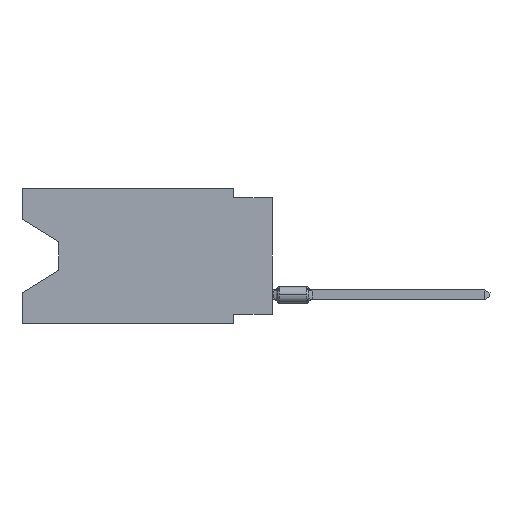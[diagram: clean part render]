
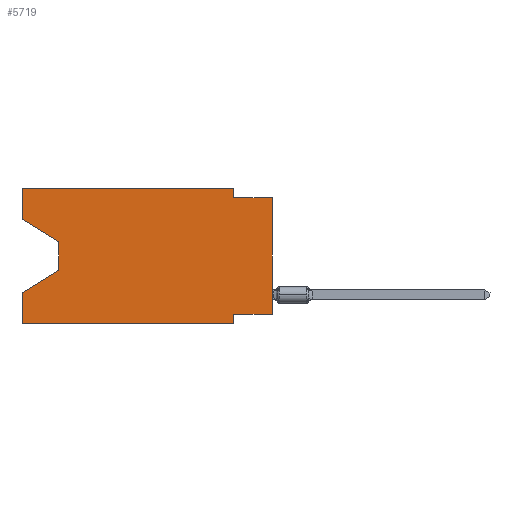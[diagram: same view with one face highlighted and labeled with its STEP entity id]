
A CAD part, left-side view. The second image highlights one B-rep face of the part: STEP entity #5719.
In plain terms, the highlighted planar face has unit normal (-1, 0, 0).
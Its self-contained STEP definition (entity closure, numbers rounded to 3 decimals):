
#72 = ORIENTED_EDGE ( 'NONE', *, *, #1886, .T. ) ;
#1260 = EDGE_CURVE ( 'NONE', #10910, #20803, #10194, .T. ) ;
#1364 = ORIENTED_EDGE ( 'NONE', *, *, #1512, .F. ) ;
#1512 = EDGE_CURVE ( 'NONE', #18159, #8420, #3695, .T. ) ;
#1534 = CARTESIAN_POINT ( 'NONE',  ( 0., 2.54, 0. ) ) ;
#1568 = ORIENTED_EDGE ( 'NONE', *, *, #5240, .T. ) ;
#1886 = EDGE_CURVE ( 'NONE', #2722, #25753, #18234, .T. ) ;
#1887 = VECTOR ( 'NONE', #8162, 1000. ) ;
#2142 = DIRECTION ( 'NONE',  ( 0., 0., 1. ) ) ;
#2150 = DIRECTION ( 'NONE',  ( 0., 0., -1. ) ) ;
#2157 = ORIENTED_EDGE ( 'NONE', *, *, #17376, .F. ) ;
#2531 = VERTEX_POINT ( 'NONE', #14428 ) ;
#2722 = VERTEX_POINT ( 'NONE', #5705 ) ;
#3095 = EDGE_CURVE ( 'NONE', #8420, #15817, #4840, .T. ) ;
#3123 = EDGE_CURVE ( 'NONE', #20083, #2722, #16212, .T. ) ;
#3695 = LINE ( 'NONE', #19400, #1887 ) ;
#3951 = EDGE_CURVE ( 'NONE', #23497, #10910, #14364, .T. ) ;
#4513 = VERTEX_POINT ( 'NONE', #12096 ) ;
#4615 = FACE_OUTER_BOUND ( 'NONE', #6433, .T. ) ;
#4840 = LINE ( 'NONE', #17813, #27555 ) ;
#4856 = CARTESIAN_POINT ( 'NONE',  ( 0., 0., 0. ) ) ;
#5065 = CARTESIAN_POINT ( 'NONE',  ( 0., 2.54, 0. ) ) ;
#5186 = CARTESIAN_POINT ( 'NONE',  ( 0., 16.383, -2.038 ) ) ;
#5240 = EDGE_CURVE ( 'NONE', #18159, #20083, #26938, .T. ) ;
#5277 = ORIENTED_EDGE ( 'NONE', *, *, #15768, .T. ) ;
#5589 = CARTESIAN_POINT ( 'NONE',  ( 0., 2.54, -8.89 ) ) ;
#5705 = CARTESIAN_POINT ( 'NONE',  ( 0., 13.97, -5.385 ) ) ;
#5719 = ADVANCED_FACE ( 'NONE', ( #4615 ), #22343, .F. ) ;
#6433 = EDGE_LOOP ( 'NONE', ( #1568, #20478, #72, #2157, #5277, #16329, #22945, #26825, #12883, #15559, #24509, #1364 ) ) ;
#6638 = VECTOR ( 'NONE', #7483, 1000. ) ;
#6887 = VECTOR ( 'NONE', #14195, 1000. ) ;
#7110 = CARTESIAN_POINT ( 'NONE',  ( 0., 2.54, -8.89 ) ) ;
#7156 = CARTESIAN_POINT ( 'NONE',  ( 0., 16.383, -6.852 ) ) ;
#7483 = DIRECTION ( 'NONE',  ( 0., -1., 0. ) ) ;
#7920 = LINE ( 'NONE', #16712, #27377 ) ;
#8162 = DIRECTION ( 'NONE',  ( 0., 0., 1. ) ) ;
#8420 = VERTEX_POINT ( 'NONE', #9087 ) ;
#9087 = CARTESIAN_POINT ( 'NONE',  ( 0., 16.383, 0. ) ) ;
#9315 = VECTOR ( 'NONE', #16072, 1000. ) ;
#9370 = VECTOR ( 'NONE', #23322, 1000. ) ;
#10067 = LINE ( 'NONE', #16417, #9370 ) ;
#10194 = LINE ( 'NONE', #5589, #25799 ) ;
#10493 = CARTESIAN_POINT ( 'NONE',  ( 0., 2.54, -8.255 ) ) ;
#10497 = EDGE_CURVE ( 'NONE', #15817, #22869, #24801, .T. ) ;
#10910 = VERTEX_POINT ( 'NONE', #10493 ) ;
#10954 = CARTESIAN_POINT ( 'NONE',  ( 0., 16.383, 0. ) ) ;
#11150 = VECTOR ( 'NONE', #20425, 1000. ) ;
#11329 = DIRECTION ( 'NONE',  ( 0., -1., 0. ) ) ;
#12096 = CARTESIAN_POINT ( 'NONE',  ( 0., 0., -0.635 ) ) ;
#12883 = ORIENTED_EDGE ( 'NONE', *, *, #14889, .F. ) ;
#13391 = VECTOR ( 'NONE', #20330, 1000. ) ;
#13849 = DIRECTION ( 'NONE',  ( 0., 0., -1. ) ) ;
#14195 = DIRECTION ( 'NONE',  ( 0., 0., -1. ) ) ;
#14364 = LINE ( 'NONE', #14644, #22070 ) ;
#14428 = CARTESIAN_POINT ( 'NONE',  ( 0., 16.383, -8.89 ) ) ;
#14644 = CARTESIAN_POINT ( 'NONE',  ( 0., 0., -8.255 ) ) ;
#14889 = EDGE_CURVE ( 'NONE', #22869, #4513, #10067, .T. ) ;
#14893 = CARTESIAN_POINT ( 'NONE',  ( 0., 0., -8.255 ) ) ;
#15445 = CARTESIAN_POINT ( 'NONE',  ( 0., 13.97, -3.505 ) ) ;
#15559 = ORIENTED_EDGE ( 'NONE', *, *, #10497, .F. ) ;
#15768 = EDGE_CURVE ( 'NONE', #2531, #20803, #18453, .T. ) ;
#15817 = VERTEX_POINT ( 'NONE', #1534 ) ;
#16072 = DIRECTION ( 'NONE',  ( 0., 0.855, -0.519 ) ) ;
#16212 = LINE ( 'NONE', #23109, #6887 ) ;
#16329 = ORIENTED_EDGE ( 'NONE', *, *, #1260, .F. ) ;
#16417 = CARTESIAN_POINT ( 'NONE',  ( 0., 0., -0.635 ) ) ;
#16712 = CARTESIAN_POINT ( 'NONE',  ( 0., 16.383, 0. ) ) ;
#17376 = EDGE_CURVE ( 'NONE', #2531, #25753, #7920, .T. ) ;
#17813 = CARTESIAN_POINT ( 'NONE',  ( 0., 16.383, 0. ) ) ;
#18159 = VERTEX_POINT ( 'NONE', #25401 ) ;
#18234 = LINE ( 'NONE', #27146, #9315 ) ;
#18258 = LINE ( 'NONE', #4856, #11150 ) ;
#18453 = LINE ( 'NONE', #25068, #6638 ) ;
#19400 = CARTESIAN_POINT ( 'NONE',  ( 0., 16.383, 0. ) ) ;
#20083 = VERTEX_POINT ( 'NONE', #15445 ) ;
#20258 = VECTOR ( 'NONE', #13849, 1000. ) ;
#20307 = CARTESIAN_POINT ( 'NONE',  ( 0., 2.54, -0.635 ) ) ;
#20330 = DIRECTION ( 'NONE',  ( 0., -0.855, -0.519 ) ) ;
#20425 = DIRECTION ( 'NONE',  ( 0., 0., 1. ) ) ;
#20478 = ORIENTED_EDGE ( 'NONE', *, *, #3123, .T. ) ;
#20803 = VERTEX_POINT ( 'NONE', #7110 ) ;
#20880 = DIRECTION ( 'NONE',  ( 0., 0., -1. ) ) ;
#21905 = DIRECTION ( 'NONE',  ( 1., 0., 0. ) ) ;
#22070 = VECTOR ( 'NONE', #25449, 1000. ) ;
#22343 = PLANE ( 'NONE',  #25680 ) ;
#22869 = VERTEX_POINT ( 'NONE', #20307 ) ;
#22945 = ORIENTED_EDGE ( 'NONE', *, *, #3951, .F. ) ;
#23109 = CARTESIAN_POINT ( 'NONE',  ( 0., 13.97, -3.505 ) ) ;
#23322 = DIRECTION ( 'NONE',  ( 0., -1., 0. ) ) ;
#23497 = VERTEX_POINT ( 'NONE', #14893 ) ;
#24509 = ORIENTED_EDGE ( 'NONE', *, *, #3095, .F. ) ;
#24801 = LINE ( 'NONE', #5065, #20258 ) ;
#25068 = CARTESIAN_POINT ( 'NONE',  ( 0., 16.383, -8.89 ) ) ;
#25401 = CARTESIAN_POINT ( 'NONE',  ( 0., 16.383, -2.038 ) ) ;
#25449 = DIRECTION ( 'NONE',  ( 0., 1., 0. ) ) ;
#25638 = EDGE_CURVE ( 'NONE', #23497, #4513, #18258, .T. ) ;
#25680 = AXIS2_PLACEMENT_3D ( 'NONE', #10954, #21905, #2150 ) ;
#25753 = VERTEX_POINT ( 'NONE', #7156 ) ;
#25799 = VECTOR ( 'NONE', #20880, 1000. ) ;
#26825 = ORIENTED_EDGE ( 'NONE', *, *, #25638, .T. ) ;
#26938 = LINE ( 'NONE', #5186, #13391 ) ;
#27146 = CARTESIAN_POINT ( 'NONE',  ( 0., 13.97, -5.385 ) ) ;
#27377 = VECTOR ( 'NONE', #2142, 1000. ) ;
#27555 = VECTOR ( 'NONE', #11329, 1000. ) ;
